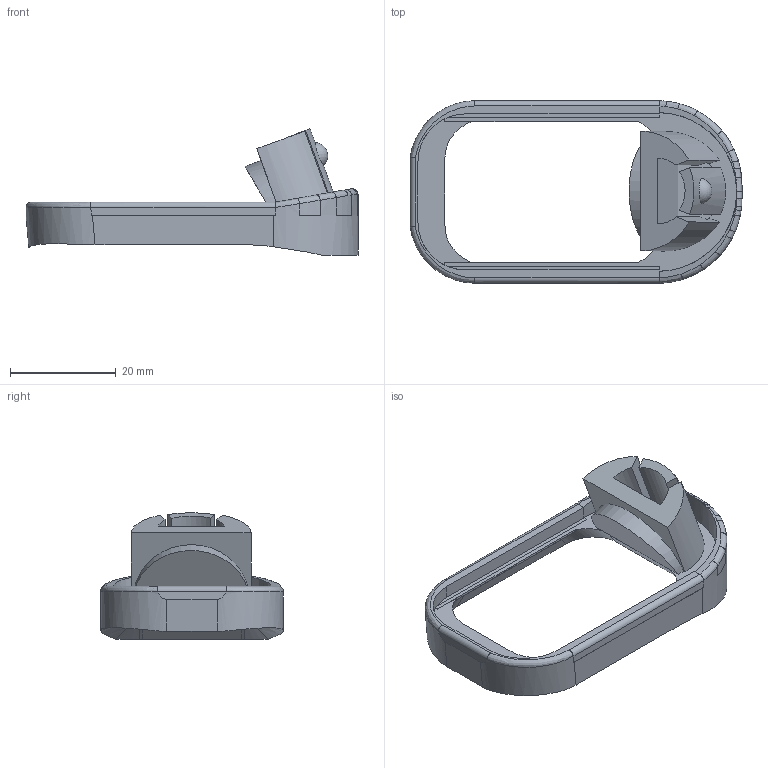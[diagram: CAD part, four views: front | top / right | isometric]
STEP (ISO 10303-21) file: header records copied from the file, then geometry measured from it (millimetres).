
FILE_DESCRIPTION(/* description */ (''),/* implementation_level */ '2;1');
FILE_NAME(/* name */ 'magwell v9.step',/* time_stamp */ '2019-12-09T23:08:12-05:00',/* author */ (''),/* organization */ (''),/* preprocessor_version */ 'ST-DEVELOPER v18',/* originating_system */ 'Autodesk Translation Framework v8.12.0.6',/* authorisation */ '');
FILE_SCHEMA (('AUTOMOTIVE_DESIGN { 1 0 10303 214 3 1 1 }'));
Length unit declared in the file: millimetre
Products named in the file (1): magwell
Bounding box: 62.71 x 34.5 x 23.83 mm (x, y, z)
Volume: 7730.5 mm3; surface area: 5613.4 mm2
Topology: 1 solids, 1 shells, 137 faces, 386 edges, 251 vertices
Faces by surface type: plane 62, bspline 50, cylinder 24, sphere 1
Entity records: 6263 total; most frequent: CARTESIAN_POINT 2971, ORIENTED_EDGE 772, DIRECTION 559, EDGE_CURVE 386, VERTEX_POINT 251, AXIS2_PLACEMENT_3D 194, LINE 171, VECTOR 171
